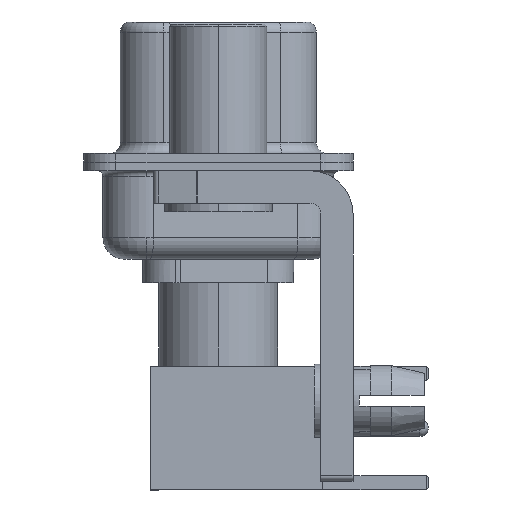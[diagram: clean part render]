
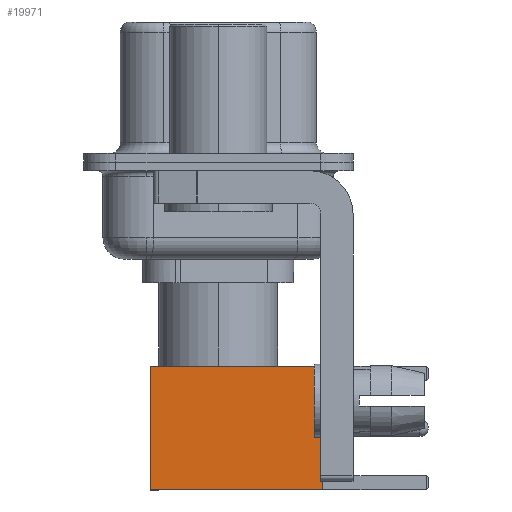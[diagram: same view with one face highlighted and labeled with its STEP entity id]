
A CAD part, left-side view. The second image highlights one B-rep face of the part: STEP entity #19971.
In plain terms, the highlighted face is planar.
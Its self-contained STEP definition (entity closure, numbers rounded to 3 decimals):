
#45 = VERTEX_POINT ( 'NONE', #515 ) ;
#515 = CARTESIAN_POINT ( 'NONE',  ( 2.875, 2.875, 8. ) ) ;
#523 = DIRECTION ( 'NONE',  ( 0., 0., -1. ) ) ;
#971 = CARTESIAN_POINT ( 'NONE',  ( -2.875, 2.875, 0. ) ) ;
#1740 = EDGE_CURVE ( 'NONE', #45, #4226, #16475, .T. ) ;
#2682 = VECTOR ( 'NONE', #523, 1000. ) ;
#4226 = VERTEX_POINT ( 'NONE', #18670 ) ;
#4482 = EDGE_CURVE ( 'NONE', #4226, #7106, #17751, .T. ) ;
#4617 = DIRECTION ( 'NONE',  ( -1., 0., 0. ) ) ;
#5185 = LINE ( 'NONE', #11643, #2682 ) ;
#6134 = CARTESIAN_POINT ( 'NONE',  ( 0., 2.875, 0. ) ) ;
#6183 = ORIENTED_EDGE ( 'NONE', *, *, #4482, .F. ) ;
#6496 = EDGE_CURVE ( 'NONE', #9111, #7106, #19967, .T. ) ;
#6573 = VECTOR ( 'NONE', #4617, 1000. ) ;
#6620 = EDGE_CURVE ( 'NONE', #45, #9111, #5185, .T. ) ;
#7106 = VERTEX_POINT ( 'NONE', #13234 ) ;
#7135 = PLANE ( 'NONE',  #12292 ) ;
#7466 = ORIENTED_EDGE ( 'NONE', *, *, #6620, .T. ) ;
#8885 = DIRECTION ( 'NONE',  ( -1., 0., 0. ) ) ;
#9111 = VERTEX_POINT ( 'NONE', #15112 ) ;
#9168 = EDGE_LOOP ( 'NONE', ( #7466, #12706, #6183, #11784 ) ) ;
#11643 = CARTESIAN_POINT ( 'NONE',  ( 2.875, 2.875, 0. ) ) ;
#11784 = ORIENTED_EDGE ( 'NONE', *, *, #1740, .F. ) ;
#11983 = CARTESIAN_POINT ( 'NONE',  ( 2.875, 2.875, 0. ) ) ;
#12081 = FACE_OUTER_BOUND ( 'NONE', #9168, .T. ) ;
#12292 = AXIS2_PLACEMENT_3D ( 'NONE', #11983, #16319, #19545 ) ;
#12706 = ORIENTED_EDGE ( 'NONE', *, *, #6496, .T. ) ;
#13234 = CARTESIAN_POINT ( 'NONE',  ( -2.875, 2.875, 0. ) ) ;
#13566 = VECTOR ( 'NONE', #18038, 1000. ) ;
#15112 = CARTESIAN_POINT ( 'NONE',  ( 2.875, 2.875, 0. ) ) ;
#16319 = DIRECTION ( 'NONE',  ( 0., 1., 0. ) ) ;
#16475 = LINE ( 'NONE', #16573, #18469 ) ;
#16573 = CARTESIAN_POINT ( 'NONE',  ( 0., 2.875, 8. ) ) ;
#17751 = LINE ( 'NONE', #971, #13566 ) ;
#18038 = DIRECTION ( 'NONE',  ( 0., 0., -1. ) ) ;
#18469 = VECTOR ( 'NONE', #8885, 1000. ) ;
#18670 = CARTESIAN_POINT ( 'NONE',  ( -2.875, 2.875, 8. ) ) ;
#19545 = DIRECTION ( 'NONE',  ( 0., 0., 1. ) ) ;
#19967 = LINE ( 'NONE', #6134, #6573 ) ;
#19971 = ADVANCED_FACE ( 'NONE', ( #12081 ), #7135, .T. ) ;
